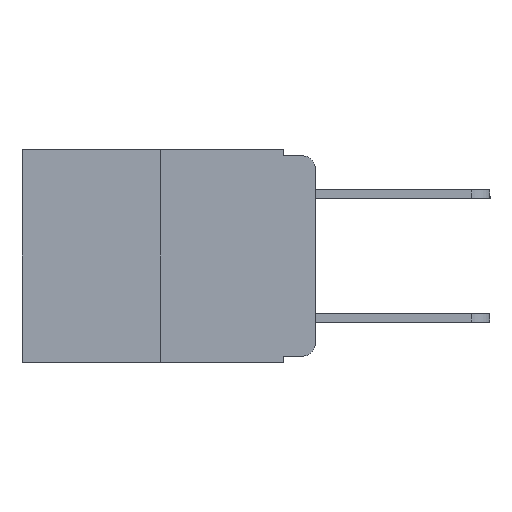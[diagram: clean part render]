
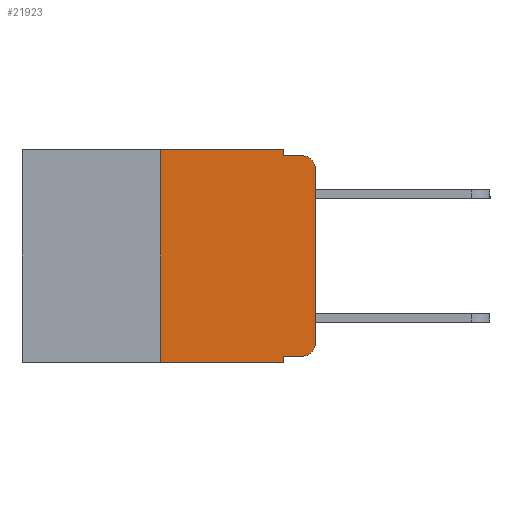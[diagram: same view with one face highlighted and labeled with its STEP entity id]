
A CAD part, left-side view. The second image highlights one B-rep face of the part: STEP entity #21923.
In plain terms, the highlighted planar face has unit normal (-1, 0, 0).
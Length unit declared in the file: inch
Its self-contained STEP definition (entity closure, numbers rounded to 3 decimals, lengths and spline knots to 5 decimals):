
#244 = DIRECTION ( 'NONE',  ( 0., 0., -1. ) ) ;
#246 = CARTESIAN_POINT ( 'NONE',  ( 0., 0.02, -0.313 ) ) ;
#449 = LINE ( 'NONE', #10371, #18324 ) ;
#1345 = LINE ( 'NONE', #5008, #19206 ) ;
#1494 = FACE_OUTER_BOUND ( 'NONE', #15058, .T. ) ;
#1633 = DIRECTION ( 'NONE',  ( 0., -1., 0. ) ) ;
#1973 = ORIENTED_EDGE ( 'NONE', *, *, #3720, .T. ) ;
#2011 = DIRECTION ( 'NONE',  ( 0., 0., -1. ) ) ;
#2090 = LINE ( 'NONE', #6579, #15921 ) ;
#2336 = DIRECTION ( 'NONE',  ( 0., 0., -1. ) ) ;
#2353 = AXIS2_PLACEMENT_3D ( 'NONE', #20961, #10659, #244 ) ;
#2517 = ORIENTED_EDGE ( 'NONE', *, *, #19265, .T. ) ;
#2816 = ORIENTED_EDGE ( 'NONE', *, *, #3159, .F. ) ;
#2841 = EDGE_CURVE ( 'NONE', #3753, #14081, #12484, .T. ) ;
#2960 = ORIENTED_EDGE ( 'NONE', *, *, #2841, .F. ) ;
#3159 = EDGE_CURVE ( 'NONE', #18626, #3753, #1345, .T. ) ;
#3277 = VECTOR ( 'NONE', #2336, 39.37008 ) ;
#3515 = ORIENTED_EDGE ( 'NONE', *, *, #4752, .T. ) ;
#3720 = EDGE_CURVE ( 'NONE', #17074, #7813, #17585, .T. ) ;
#3753 = VERTEX_POINT ( 'NONE', #7845 ) ;
#3775 = DIRECTION ( 'NONE',  ( 0., 0., 1. ) ) ;
#4180 = CARTESIAN_POINT ( 'NONE',  ( 0., 0.051, -0.333 ) ) ;
#4362 = CIRCLE ( 'NONE', #2353, 0.02 ) ;
#4561 = LINE ( 'NONE', #4180, #21299 ) ;
#4747 = EDGE_CURVE ( 'NONE', #14081, #16158, #449, .T. ) ;
#4752 = EDGE_CURVE ( 'NONE', #8371, #8058, #14296, .T. ) ;
#5008 = CARTESIAN_POINT ( 'NONE',  ( 0., 0.473, 0. ) ) ;
#5945 = DIRECTION ( 'NONE',  ( 0., -1., 0. ) ) ;
#6579 = CARTESIAN_POINT ( 'NONE',  ( 0., 0.051, 0. ) ) ;
#6825 = CARTESIAN_POINT ( 'NONE',  ( 0., 0., -0.03 ) ) ;
#7097 = CARTESIAN_POINT ( 'NONE',  ( 0., 0., 0. ) ) ;
#7402 = DIRECTION ( 'NONE',  ( 0., 0., 1. ) ) ;
#7813 = VERTEX_POINT ( 'NONE', #6825 ) ;
#7845 = CARTESIAN_POINT ( 'NONE',  ( 0., 0.051, 0. ) ) ;
#8058 = VERTEX_POINT ( 'NONE', #16091 ) ;
#8207 = ORIENTED_EDGE ( 'NONE', *, *, #13114, .F. ) ;
#8227 = ORIENTED_EDGE ( 'NONE', *, *, #20403, .T. ) ;
#8371 = VERTEX_POINT ( 'NONE', #9945 ) ;
#8469 = ORIENTED_EDGE ( 'NONE', *, *, #4747, .F. ) ;
#8553 = CARTESIAN_POINT ( 'NONE',  ( 0., 0.051, 0. ) ) ;
#9488 = DIRECTION ( 'NONE',  ( 1., 0., 0. ) ) ;
#9945 = CARTESIAN_POINT ( 'NONE',  ( 0., 0.25, -0.343 ) ) ;
#10147 = ORIENTED_EDGE ( 'NONE', *, *, #11418, .T. ) ;
#10249 = CARTESIAN_POINT ( 'NONE',  ( 0., 0.051, -0.333 ) ) ;
#10371 = CARTESIAN_POINT ( 'NONE',  ( 0., 0.051, -0.01 ) ) ;
#10659 = DIRECTION ( 'NONE',  ( -1., 0., 0. ) ) ;
#11029 = VERTEX_POINT ( 'NONE', #16581 ) ;
#11123 = LINE ( 'NONE', #15994, #15201 ) ;
#11418 = EDGE_CURVE ( 'NONE', #7813, #16158, #4362, .T. ) ;
#12240 = DIRECTION ( 'NONE',  ( 0., -1., 0. ) ) ;
#12388 = DIRECTION ( 'NONE',  ( -1., 0., 0. ) ) ;
#12484 = LINE ( 'NONE', #8553, #3277 ) ;
#12531 = VERTEX_POINT ( 'NONE', #10249 ) ;
#12703 = CARTESIAN_POINT ( 'NONE',  ( 0., 0.051, -0.01 ) ) ;
#12829 = CARTESIAN_POINT ( 'NONE',  ( 0., 0.25, 0. ) ) ;
#13114 = EDGE_CURVE ( 'NONE', #12531, #8058, #2090, .T. ) ;
#14081 = VERTEX_POINT ( 'NONE', #12703 ) ;
#14296 = LINE ( 'NONE', #20600, #14841 ) ;
#14651 = PLANE ( 'NONE',  #22062 ) ;
#14841 = VECTOR ( 'NONE', #1633, 39.37008 ) ;
#15058 = EDGE_LOOP ( 'NONE', ( #1973, #10147, #8469, #2960, #2816, #18484, #3515, #8207, #2517, #8227 ) ) ;
#15201 = VECTOR ( 'NONE', #7402, 39.37008 ) ;
#15921 = VECTOR ( 'NONE', #18623, 39.37008 ) ;
#15994 = CARTESIAN_POINT ( 'NONE',  ( 0., 0.25, 0. ) ) ;
#16091 = CARTESIAN_POINT ( 'NONE',  ( 0., 0.051, -0.343 ) ) ;
#16158 = VERTEX_POINT ( 'NONE', #16217 ) ;
#16194 = AXIS2_PLACEMENT_3D ( 'NONE', #246, #12388, #2011 ) ;
#16217 = CARTESIAN_POINT ( 'NONE',  ( 0., 0.02, -0.01 ) ) ;
#16581 = CARTESIAN_POINT ( 'NONE',  ( 0., 0.02, -0.333 ) ) ;
#17074 = VERTEX_POINT ( 'NONE', #17306 ) ;
#17306 = CARTESIAN_POINT ( 'NONE',  ( 0., 0., -0.313 ) ) ;
#17585 = LINE ( 'NONE', #7097, #21570 ) ;
#17835 = EDGE_CURVE ( 'NONE', #8371, #18626, #11123, .T. ) ;
#18100 = CARTESIAN_POINT ( 'NONE',  ( 0., 0.473, 0. ) ) ;
#18324 = VECTOR ( 'NONE', #12240, 39.37008 ) ;
#18472 = DIRECTION ( 'NONE',  ( 0., -1., 0. ) ) ;
#18484 = ORIENTED_EDGE ( 'NONE', *, *, #17835, .F. ) ;
#18623 = DIRECTION ( 'NONE',  ( 0., 0., -1. ) ) ;
#18626 = VERTEX_POINT ( 'NONE', #12829 ) ;
#19206 = VECTOR ( 'NONE', #18472, 39.37008 ) ;
#19265 = EDGE_CURVE ( 'NONE', #12531, #11029, #4561, .T. ) ;
#19924 = CIRCLE ( 'NONE', #16194, 0.02 ) ;
#20403 = EDGE_CURVE ( 'NONE', #11029, #17074, #19924, .T. ) ;
#20600 = CARTESIAN_POINT ( 'NONE',  ( 0., 0.473, -0.343 ) ) ;
#20961 = CARTESIAN_POINT ( 'NONE',  ( 0., 0.02, -0.03 ) ) ;
#21299 = VECTOR ( 'NONE', #5945, 39.37008 ) ;
#21522 = DIRECTION ( 'NONE',  ( 0., 0., -1. ) ) ;
#21570 = VECTOR ( 'NONE', #3775, 39.37008 ) ;
#21923 = ADVANCED_FACE ( 'NONE', ( #1494 ), #14651, .F. ) ;
#22062 = AXIS2_PLACEMENT_3D ( 'NONE', #18100, #9488, #21522 ) ;
